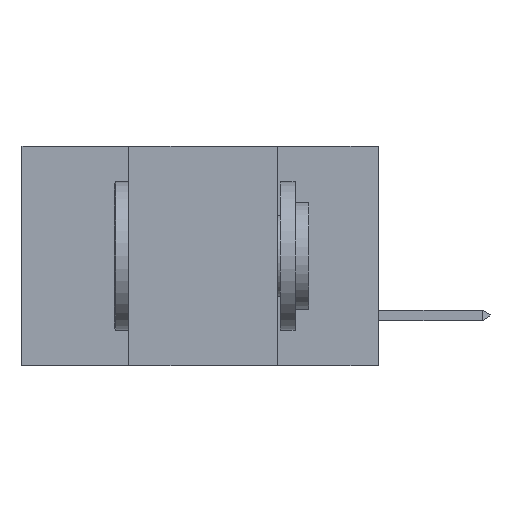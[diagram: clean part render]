
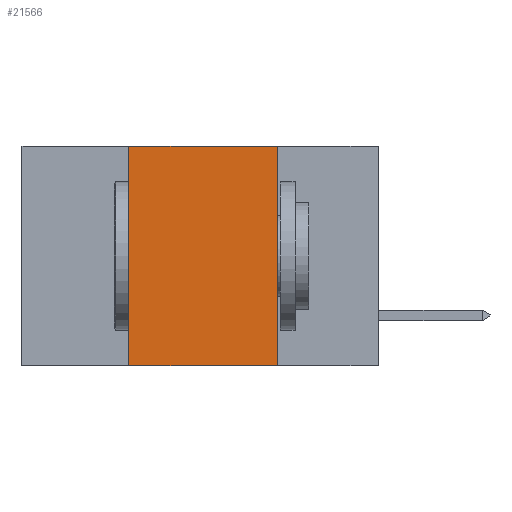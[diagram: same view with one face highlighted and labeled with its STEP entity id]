
A CAD part, left-side view. The second image highlights one B-rep face of the part: STEP entity #21566.
In plain terms, the highlighted planar face has unit normal (-1, 0, 0).
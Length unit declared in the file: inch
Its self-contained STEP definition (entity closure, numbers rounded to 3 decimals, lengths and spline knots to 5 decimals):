
#568 = EDGE_CURVE ( 'NONE', #19707, #19347, #6277, .T. ) ;
#1238 = DIRECTION ( 'NONE',  ( 0., -1., 0. ) ) ;
#1531 = ORIENTED_EDGE ( 'NONE', *, *, #2143, .F. ) ;
#1623 = LINE ( 'NONE', #10709, #21293 ) ;
#1737 = CARTESIAN_POINT ( 'NONE',  ( 0., 0.42, -0.37 ) ) ;
#2143 = EDGE_CURVE ( 'NONE', #2755, #12268, #1623, .T. ) ;
#2755 = VERTEX_POINT ( 'NONE', #13174 ) ;
#3292 = ORIENTED_EDGE ( 'NONE', *, *, #568, .F. ) ;
#4268 = DIRECTION ( 'NONE',  ( 0., 0., -1. ) ) ;
#6062 = EDGE_CURVE ( 'NONE', #19347, #2755, #11370, .T. ) ;
#6277 = LINE ( 'NONE', #8389, #19252 ) ;
#8389 = CARTESIAN_POINT ( 'NONE',  ( 0., 0.42, 0. ) ) ;
#8905 = AXIS2_PLACEMENT_3D ( 'NONE', #16245, #12774, #4268 ) ;
#9698 = CARTESIAN_POINT ( 'NONE',  ( 0., 0.6, -0.37 ) ) ;
#9713 = VECTOR ( 'NONE', #17911, 39.37008 ) ;
#10129 = CARTESIAN_POINT ( 'NONE',  ( 0., 0.17, -0.37 ) ) ;
#10709 = CARTESIAN_POINT ( 'NONE',  ( 0., 0.17, 0. ) ) ;
#10935 = EDGE_LOOP ( 'NONE', ( #1531, #21158, #3292, #18803 ) ) ;
#11001 = DIRECTION ( 'NONE',  ( 0., 0., -1. ) ) ;
#11370 = LINE ( 'NONE', #12613, #9713 ) ;
#11504 = LINE ( 'NONE', #9698, #13921 ) ;
#11852 = EDGE_CURVE ( 'NONE', #19707, #12268, #11504, .T. ) ;
#12268 = VERTEX_POINT ( 'NONE', #10129 ) ;
#12613 = CARTESIAN_POINT ( 'NONE',  ( 0., 0.6, 0. ) ) ;
#12774 = DIRECTION ( 'NONE',  ( 1., 0., 0. ) ) ;
#13174 = CARTESIAN_POINT ( 'NONE',  ( 0., 0.17, 0. ) ) ;
#13921 = VECTOR ( 'NONE', #1238, 39.37008 ) ;
#16245 = CARTESIAN_POINT ( 'NONE',  ( 0., 0.6, 0. ) ) ;
#16394 = PLANE ( 'NONE',  #8905 ) ;
#16584 = CARTESIAN_POINT ( 'NONE',  ( 0., 0.42, 0. ) ) ;
#17911 = DIRECTION ( 'NONE',  ( 0., -1., 0. ) ) ;
#18803 = ORIENTED_EDGE ( 'NONE', *, *, #11852, .T. ) ;
#19252 = VECTOR ( 'NONE', #22053, 39.37008 ) ;
#19325 = FACE_OUTER_BOUND ( 'NONE', #10935, .T. ) ;
#19347 = VERTEX_POINT ( 'NONE', #16584 ) ;
#19707 = VERTEX_POINT ( 'NONE', #1737 ) ;
#21158 = ORIENTED_EDGE ( 'NONE', *, *, #6062, .F. ) ;
#21293 = VECTOR ( 'NONE', #11001, 39.37008 ) ;
#21566 = ADVANCED_FACE ( 'NONE', ( #19325 ), #16394, .F. ) ;
#22053 = DIRECTION ( 'NONE',  ( 0., 0., 1. ) ) ;
